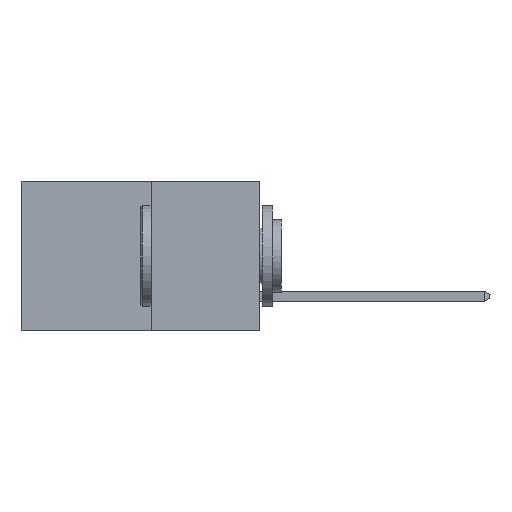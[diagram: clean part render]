
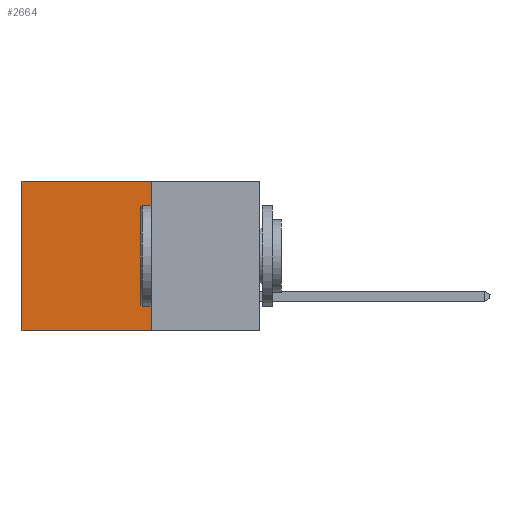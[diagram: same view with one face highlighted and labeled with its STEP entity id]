
A CAD part, left-side view. The second image highlights one B-rep face of the part: STEP entity #2664.
In plain terms, the highlighted planar face has unit normal (-1, 0, 0).
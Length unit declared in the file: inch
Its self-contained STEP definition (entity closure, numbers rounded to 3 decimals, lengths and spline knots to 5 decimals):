
#775 = VERTEX_POINT ( 'NONE', #833 ) ;
#833 = CARTESIAN_POINT ( 'NONE',  ( 0.277, 0.59, -0.37 ) ) ;
#1604 = DIRECTION ( 'NONE',  ( 0., 1., 0. ) ) ;
#1665 = ORIENTED_EDGE ( 'NONE', *, *, #3601, .F. ) ;
#2664 = ADVANCED_FACE ( 'NONE', ( #3267 ), #13012, .F. ) ;
#3267 = FACE_OUTER_BOUND ( 'NONE', #7148, .T. ) ;
#3592 = VECTOR ( 'NONE', #1604, 39.37008 ) ;
#3601 = EDGE_CURVE ( 'NONE', #5595, #7202, #14022, .T. ) ;
#3750 = VECTOR ( 'NONE', #4606, 39.37008 ) ;
#4115 = CARTESIAN_POINT ( 'NONE',  ( 0.277, 0.27, 0. ) ) ;
#4606 = DIRECTION ( 'NONE',  ( 0., 0., -1. ) ) ;
#5148 = CARTESIAN_POINT ( 'NONE',  ( 0.277, 0.27, -0.37 ) ) ;
#5403 = VECTOR ( 'NONE', #16631, 39.37008 ) ;
#5595 = VERTEX_POINT ( 'NONE', #4115 ) ;
#6111 = EDGE_CURVE ( 'NONE', #7202, #775, #16992, .T. ) ;
#6415 = VERTEX_POINT ( 'NONE', #27965 ) ;
#7148 = EDGE_LOOP ( 'NONE', ( #10325, #25480, #1665, #7779 ) ) ;
#7202 = VERTEX_POINT ( 'NONE', #12762 ) ;
#7779 = ORIENTED_EDGE ( 'NONE', *, *, #21796, .T. ) ;
#9311 = DIRECTION ( 'NONE',  ( 1., 0., 0. ) ) ;
#9453 = LINE ( 'NONE', #25490, #3592 ) ;
#10325 = ORIENTED_EDGE ( 'NONE', *, *, #14665, .T. ) ;
#10456 = DIRECTION ( 'NONE',  ( 0., 0., -1. ) ) ;
#12762 = CARTESIAN_POINT ( 'NONE',  ( 0.277, 0.27, -0.37 ) ) ;
#13012 = PLANE ( 'NONE',  #15826 ) ;
#14022 = LINE ( 'NONE', #5148, #3750 ) ;
#14662 = LINE ( 'NONE', #21158, #25448 ) ;
#14665 = EDGE_CURVE ( 'NONE', #6415, #775, #14662, .T. ) ;
#14747 = CARTESIAN_POINT ( 'NONE',  ( 0.277, 0.27, -0.37 ) ) ;
#15826 = AXIS2_PLACEMENT_3D ( 'NONE', #21477, #9311, #10456 ) ;
#16631 = DIRECTION ( 'NONE',  ( 0., 1., 0. ) ) ;
#16992 = LINE ( 'NONE', #14747, #5403 ) ;
#21158 = CARTESIAN_POINT ( 'NONE',  ( 0.277, 0.59, -0.37 ) ) ;
#21477 = CARTESIAN_POINT ( 'NONE',  ( 0.277, 0.27, -0.37 ) ) ;
#21796 = EDGE_CURVE ( 'NONE', #5595, #6415, #9453, .T. ) ;
#23243 = DIRECTION ( 'NONE',  ( 0., 0., -1. ) ) ;
#25448 = VECTOR ( 'NONE', #23243, 39.37008 ) ;
#25480 = ORIENTED_EDGE ( 'NONE', *, *, #6111, .F. ) ;
#25490 = CARTESIAN_POINT ( 'NONE',  ( 0.277, 0.27, 0. ) ) ;
#27965 = CARTESIAN_POINT ( 'NONE',  ( 0.277, 0.59, 0. ) ) ;
